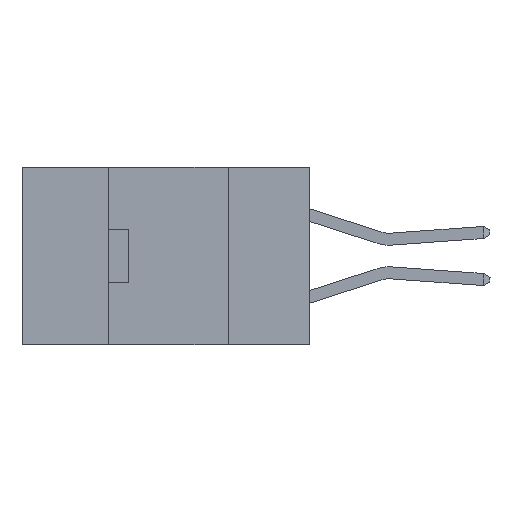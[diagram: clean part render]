
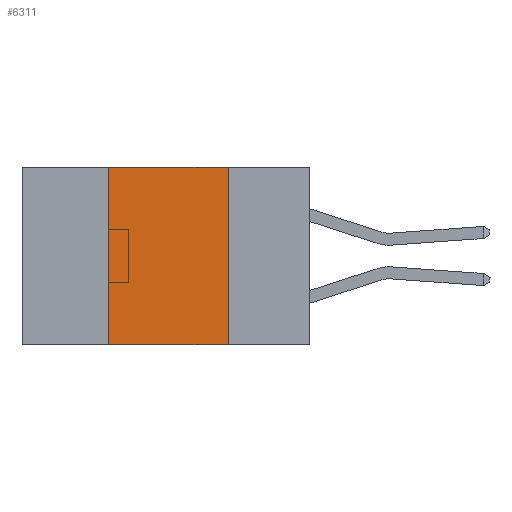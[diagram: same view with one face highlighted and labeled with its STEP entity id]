
A CAD part, left-side view. The second image highlights one B-rep face of the part: STEP entity #6311.
In plain terms, the highlighted planar face has unit normal (-1, 0, 0).
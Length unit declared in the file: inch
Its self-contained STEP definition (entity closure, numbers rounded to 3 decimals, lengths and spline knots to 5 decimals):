
#2220 = LINE ( 'NONE', #20299, #13583 ) ;
#3422 = CARTESIAN_POINT ( 'NONE',  ( 0., 0.17, -0.37 ) ) ;
#3570 = EDGE_CURVE ( 'NONE', #14932, #12084, #25282, .T. ) ;
#4254 = CARTESIAN_POINT ( 'NONE',  ( 0., 0.42, 0. ) ) ;
#4538 = DIRECTION ( 'NONE',  ( 1., 0., 0. ) ) ;
#5706 = DIRECTION ( 'NONE',  ( 0., 0., -1. ) ) ;
#6311 = ADVANCED_FACE ( 'NONE', ( #12815 ), #18030, .F. ) ;
#7483 = VECTOR ( 'NONE', #17511, 39.37008 ) ;
#7822 = CARTESIAN_POINT ( 'NONE',  ( 0., 0.42, -0.37 ) ) ;
#9777 = LINE ( 'NONE', #3422, #20962 ) ;
#11448 = DIRECTION ( 'NONE',  ( 0., 0., 1. ) ) ;
#12084 = VERTEX_POINT ( 'NONE', #12817 ) ;
#12815 = FACE_OUTER_BOUND ( 'NONE', #14780, .T. ) ;
#12817 = CARTESIAN_POINT ( 'NONE',  ( 0., 0.17, 0. ) ) ;
#13028 = CARTESIAN_POINT ( 'NONE',  ( 0., 0.6, 0. ) ) ;
#13259 = VECTOR ( 'NONE', #14040, 39.37008 ) ;
#13583 = VECTOR ( 'NONE', #11448, 39.37008 ) ;
#14040 = DIRECTION ( 'NONE',  ( 0., -1., 0. ) ) ;
#14780 = EDGE_LOOP ( 'NONE', ( #18801, #19944, #25122, #18439 ) ) ;
#14932 = VERTEX_POINT ( 'NONE', #4254 ) ;
#15284 = VERTEX_POINT ( 'NONE', #7822 ) ;
#15304 = EDGE_CURVE ( 'NONE', #12084, #28958, #9777, .T. ) ;
#16232 = EDGE_CURVE ( 'NONE', #15284, #14932, #2220, .T. ) ;
#17511 = DIRECTION ( 'NONE',  ( 0., -1., 0. ) ) ;
#17935 = CARTESIAN_POINT ( 'NONE',  ( 0., 0.6, 0. ) ) ;
#18030 = PLANE ( 'NONE',  #23304 ) ;
#18439 = ORIENTED_EDGE ( 'NONE', *, *, #19780, .T. ) ;
#18480 = LINE ( 'NONE', #27305, #13259 ) ;
#18801 = ORIENTED_EDGE ( 'NONE', *, *, #15304, .F. ) ;
#19328 = CARTESIAN_POINT ( 'NONE',  ( 0., 0.17, -0.37 ) ) ;
#19780 = EDGE_CURVE ( 'NONE', #15284, #28958, #18480, .T. ) ;
#19944 = ORIENTED_EDGE ( 'NONE', *, *, #3570, .F. ) ;
#20264 = DIRECTION ( 'NONE',  ( 0., 0., -1. ) ) ;
#20299 = CARTESIAN_POINT ( 'NONE',  ( 0., 0.42, -0.37 ) ) ;
#20962 = VECTOR ( 'NONE', #5706, 39.37008 ) ;
#23304 = AXIS2_PLACEMENT_3D ( 'NONE', #17935, #4538, #20264 ) ;
#25122 = ORIENTED_EDGE ( 'NONE', *, *, #16232, .F. ) ;
#25282 = LINE ( 'NONE', #13028, #7483 ) ;
#27305 = CARTESIAN_POINT ( 'NONE',  ( 0., 0.6, -0.37 ) ) ;
#28958 = VERTEX_POINT ( 'NONE', #19328 ) ;
